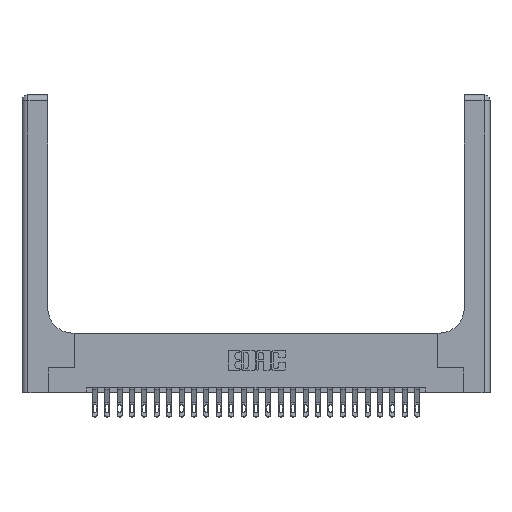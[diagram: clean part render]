
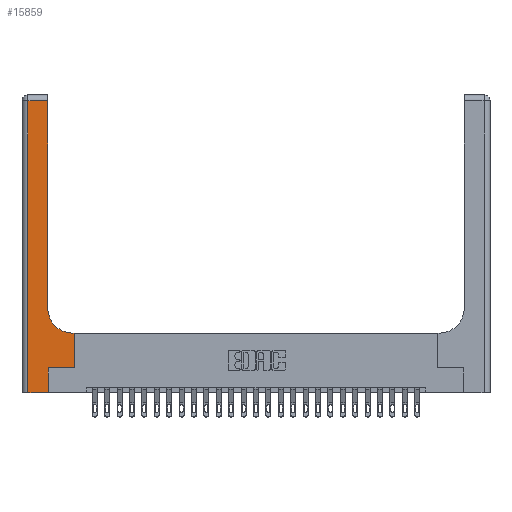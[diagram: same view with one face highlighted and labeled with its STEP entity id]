
A CAD part, top view. The second image highlights one B-rep face of the part: STEP entity #15859.
In plain terms, the highlighted planar face has unit normal (0, 0, 1).
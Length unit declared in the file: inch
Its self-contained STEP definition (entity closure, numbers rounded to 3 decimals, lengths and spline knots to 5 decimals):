
#181 = CARTESIAN_POINT ( 'NONE',  ( 0.265, 0.25, 0.37 ) ) ;
#348 = DIRECTION ( 'NONE',  ( 0., 1., 0. ) ) ;
#475 = CARTESIAN_POINT ( 'NONE',  ( 0.26, 3., 0.37 ) ) ;
#525 = DIRECTION ( 'NONE',  ( 1., 0., 0. ) ) ;
#1140 = DIRECTION ( 'NONE',  ( -1., 0., 0. ) ) ;
#1270 = EDGE_CURVE ( 'NONE', #24638, #12356, #9208, .T. ) ;
#1394 = PLANE ( 'NONE',  #25532 ) ;
#1577 = DIRECTION ( 'NONE',  ( -1., 0., 0. ) ) ;
#1791 = VERTEX_POINT ( 'NONE', #16109 ) ;
#3326 = ORIENTED_EDGE ( 'NONE', *, *, #3616, .T. ) ;
#3585 = VERTEX_POINT ( 'NONE', #14262 ) ;
#3616 = EDGE_CURVE ( 'NONE', #12222, #22205, #4797, .T. ) ;
#3990 = VECTOR ( 'NONE', #11961, 39.37008 ) ;
#4058 = VECTOR ( 'NONE', #7739, 39.37008 ) ;
#4265 = ORIENTED_EDGE ( 'NONE', *, *, #17121, .T. ) ;
#4681 = CARTESIAN_POINT ( 'NONE',  ( 0.06, 0., 0.37 ) ) ;
#4797 = LINE ( 'NONE', #18282, #19273 ) ;
#5243 = LINE ( 'NONE', #12880, #15860 ) ;
#5524 = LINE ( 'NONE', #9442, #4058 ) ;
#5676 = CARTESIAN_POINT ( 'NONE',  ( 0.26, 0.85, 0.37 ) ) ;
#5920 = AXIS2_PLACEMENT_3D ( 'NONE', #23755, #11832, #19607 ) ;
#6950 = VERTEX_POINT ( 'NONE', #23714 ) ;
#7404 = LINE ( 'NONE', #25294, #22578 ) ;
#7435 = ORIENTED_EDGE ( 'NONE', *, *, #12363, .T. ) ;
#7564 = VERTEX_POINT ( 'NONE', #21169 ) ;
#7739 = DIRECTION ( 'NONE',  ( 0., 1., 0. ) ) ;
#8112 = EDGE_CURVE ( 'NONE', #6950, #7564, #15308, .T. ) ;
#8633 = VERTEX_POINT ( 'NONE', #5676 ) ;
#9053 = DIRECTION ( 'NONE',  ( 0., 0., -1. ) ) ;
#9130 = VECTOR ( 'NONE', #1577, 39.37008 ) ;
#9154 = EDGE_CURVE ( 'NONE', #1791, #8633, #14599, .T. ) ;
#9208 = LINE ( 'NONE', #18790, #15452 ) ;
#9442 = CARTESIAN_POINT ( 'NONE',  ( 0.265, 0., 0.37 ) ) ;
#10513 = ORIENTED_EDGE ( 'NONE', *, *, #25140, .T. ) ;
#11292 = CARTESIAN_POINT ( 'NONE',  ( 0., 2.94, 0.37 ) ) ;
#11832 = DIRECTION ( 'NONE',  ( 0., 0., -1. ) ) ;
#11961 = DIRECTION ( 'NONE',  ( 1., 0., 0. ) ) ;
#12059 = VECTOR ( 'NONE', #348, 39.37008 ) ;
#12135 = CARTESIAN_POINT ( 'NONE',  ( 0.528, 0.25, 0.37 ) ) ;
#12222 = VERTEX_POINT ( 'NONE', #4681 ) ;
#12356 = VERTEX_POINT ( 'NONE', #23341 ) ;
#12363 = EDGE_CURVE ( 'NONE', #12356, #1791, #7404, .T. ) ;
#12880 = CARTESIAN_POINT ( 'NONE',  ( 0.06, 3., 0.37 ) ) ;
#13202 = EDGE_CURVE ( 'NONE', #3585, #24638, #21831, .T. ) ;
#14262 = CARTESIAN_POINT ( 'NONE',  ( 0.265, 0.25, 0.37 ) ) ;
#14599 = CIRCLE ( 'NONE', #5920, 0.25 ) ;
#15308 = LINE ( 'NONE', #11292, #9130 ) ;
#15452 = VECTOR ( 'NONE', #24617, 39.37008 ) ;
#15859 = ADVANCED_FACE ( 'NONE', ( #17075 ), #1394, .F. ) ;
#15860 = VECTOR ( 'NONE', #21041, 39.37008 ) ;
#16109 = CARTESIAN_POINT ( 'NONE',  ( 0.51, 0.6, 0.37 ) ) ;
#16513 = ORIENTED_EDGE ( 'NONE', *, *, #13202, .T. ) ;
#17075 = FACE_OUTER_BOUND ( 'NONE', #17906, .T. ) ;
#17121 = EDGE_CURVE ( 'NONE', #22205, #3585, #5524, .T. ) ;
#17259 = DIRECTION ( 'NONE',  ( -1., 0., 0. ) ) ;
#17906 = EDGE_LOOP ( 'NONE', ( #22585, #23717, #10513, #3326, #4265, #16513, #23877, #7435, #23321 ) ) ;
#18282 = CARTESIAN_POINT ( 'NONE',  ( 0., 0., 0.37 ) ) ;
#18790 = CARTESIAN_POINT ( 'NONE',  ( 0.528, 0.25, 0.37 ) ) ;
#19273 = VECTOR ( 'NONE', #525, 39.37008 ) ;
#19607 = DIRECTION ( 'NONE',  ( 1., 0., 0. ) ) ;
#19877 = CARTESIAN_POINT ( 'NONE',  ( 0.265, 0., 0.37 ) ) ;
#21041 = DIRECTION ( 'NONE',  ( 0., -1., 0. ) ) ;
#21169 = CARTESIAN_POINT ( 'NONE',  ( 0.06, 2.94, 0.37 ) ) ;
#21831 = LINE ( 'NONE', #181, #3990 ) ;
#22205 = VERTEX_POINT ( 'NONE', #19877 ) ;
#22578 = VECTOR ( 'NONE', #17259, 39.37008 ) ;
#22585 = ORIENTED_EDGE ( 'NONE', *, *, #23316, .T. ) ;
#23316 = EDGE_CURVE ( 'NONE', #8633, #6950, #24443, .T. ) ;
#23321 = ORIENTED_EDGE ( 'NONE', *, *, #9154, .T. ) ;
#23341 = CARTESIAN_POINT ( 'NONE',  ( 0.528, 0.6, 0.37 ) ) ;
#23714 = CARTESIAN_POINT ( 'NONE',  ( 0.26, 2.94, 0.37 ) ) ;
#23717 = ORIENTED_EDGE ( 'NONE', *, *, #8112, .T. ) ;
#23755 = CARTESIAN_POINT ( 'NONE',  ( 0.51, 0.85, 0.37 ) ) ;
#23877 = ORIENTED_EDGE ( 'NONE', *, *, #1270, .T. ) ;
#24443 = LINE ( 'NONE', #475, #12059 ) ;
#24617 = DIRECTION ( 'NONE',  ( 0., 1., 0. ) ) ;
#24638 = VERTEX_POINT ( 'NONE', #12135 ) ;
#24857 = CARTESIAN_POINT ( 'NONE',  ( 0., 3., 0.37 ) ) ;
#25140 = EDGE_CURVE ( 'NONE', #7564, #12222, #5243, .T. ) ;
#25294 = CARTESIAN_POINT ( 'NONE',  ( 0.26, 0.6, 0.37 ) ) ;
#25532 = AXIS2_PLACEMENT_3D ( 'NONE', #24857, #9053, #1140 ) ;
